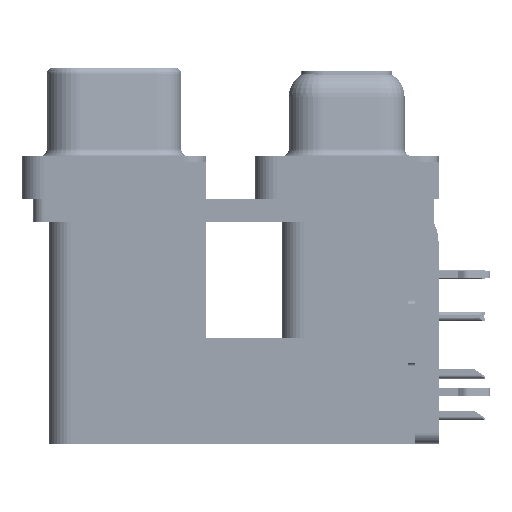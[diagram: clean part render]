
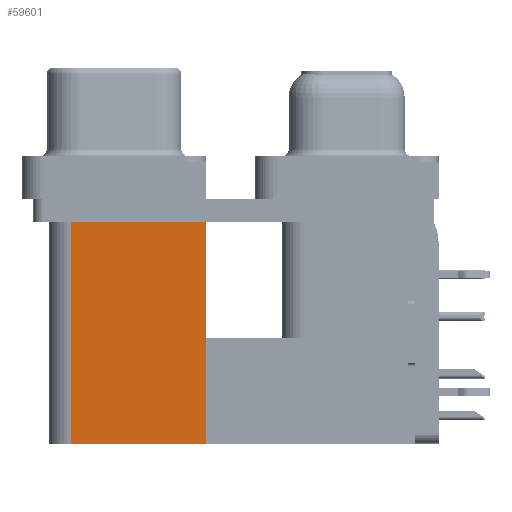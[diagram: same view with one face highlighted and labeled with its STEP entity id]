
A CAD part, left-side view. The second image highlights one B-rep face of the part: STEP entity #59601.
In plain terms, the highlighted planar face has unit normal (-1, 0, 0).
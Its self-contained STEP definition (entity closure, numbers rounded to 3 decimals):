
#302 = DIRECTION ( 'NONE',  ( 0., 0., -1. ) ) ;
#499 = DIRECTION ( 'NONE',  ( 0., 0., 1. ) ) ;
#2884 = CARTESIAN_POINT ( 'NONE',  ( 3.79, 9.6, -19.2 ) ) ;
#4063 = DIRECTION ( 'NONE',  ( 0., 1., 0. ) ) ;
#15780 = CARTESIAN_POINT ( 'NONE',  ( 3.79, 9.6, -2.5 ) ) ;
#16075 = CARTESIAN_POINT ( 'NONE',  ( 3.79, 9.6, -19.2 ) ) ;
#16296 = AXIS2_PLACEMENT_3D ( 'NONE', #53029, #54420, #302 ) ;
#16870 = LINE ( 'NONE', #29296, #69926 ) ;
#19314 = EDGE_CURVE ( 'NONE', #41306, #42889, #16870, .T. ) ;
#24977 = EDGE_LOOP ( 'NONE', ( #25129, #46414, #40945, #28522 ) ) ;
#25129 = ORIENTED_EDGE ( 'NONE', *, *, #42823, .T. ) ;
#27101 = DIRECTION ( 'NONE',  ( 0., 1., 0. ) ) ;
#28522 = ORIENTED_EDGE ( 'NONE', *, *, #50898, .T. ) ;
#29296 = CARTESIAN_POINT ( 'NONE',  ( 3.79, 18.8, -19.2 ) ) ;
#35881 = CARTESIAN_POINT ( 'NONE',  ( 3.79, 18.8, -19.2 ) ) ;
#39275 = EDGE_CURVE ( 'NONE', #58003, #41306, #49542, .T. ) ;
#39897 = DIRECTION ( 'NONE',  ( 0., 0., 1. ) ) ;
#40945 = ORIENTED_EDGE ( 'NONE', *, *, #39275, .F. ) ;
#41306 = VERTEX_POINT ( 'NONE', #35881 ) ;
#42679 = PLANE ( 'NONE',  #16296 ) ;
#42823 = EDGE_CURVE ( 'NONE', #43924, #42889, #48184, .T. ) ;
#42889 = VERTEX_POINT ( 'NONE', #59919 ) ;
#43924 = VERTEX_POINT ( 'NONE', #52155 ) ;
#45234 = LINE ( 'NONE', #2884, #52073 ) ;
#45643 = CARTESIAN_POINT ( 'NONE',  ( 3.79, 9.6, -19.2 ) ) ;
#46414 = ORIENTED_EDGE ( 'NONE', *, *, #19314, .F. ) ;
#48184 = LINE ( 'NONE', #15780, #48359 ) ;
#48359 = VECTOR ( 'NONE', #4063, 1000. ) ;
#49542 = LINE ( 'NONE', #16075, #65064 ) ;
#50898 = EDGE_CURVE ( 'NONE', #58003, #43924, #45234, .T. ) ;
#52073 = VECTOR ( 'NONE', #39897, 1000. ) ;
#52155 = CARTESIAN_POINT ( 'NONE',  ( 3.79, 9.6, -2.5 ) ) ;
#53029 = CARTESIAN_POINT ( 'NONE',  ( 3.79, 9.6, -19.2 ) ) ;
#54420 = DIRECTION ( 'NONE',  ( 1., 0., 0. ) ) ;
#58003 = VERTEX_POINT ( 'NONE', #45643 ) ;
#58358 = FACE_OUTER_BOUND ( 'NONE', #24977, .T. ) ;
#59601 = ADVANCED_FACE ( 'NONE', ( #58358 ), #42679, .F. ) ;
#59919 = CARTESIAN_POINT ( 'NONE',  ( 3.79, 18.8, -2.5 ) ) ;
#65064 = VECTOR ( 'NONE', #27101, 1000. ) ;
#69926 = VECTOR ( 'NONE', #499, 1000. ) ;
